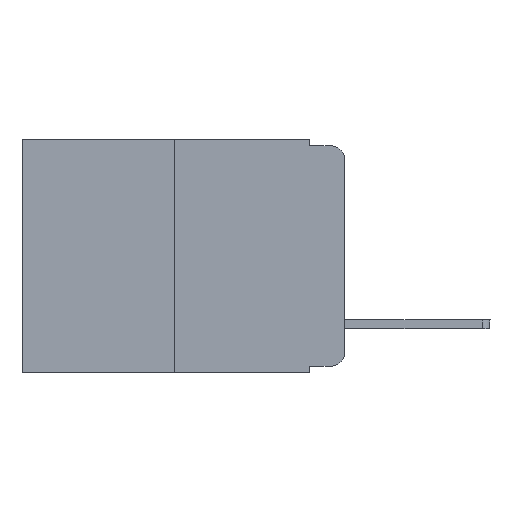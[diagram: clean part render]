
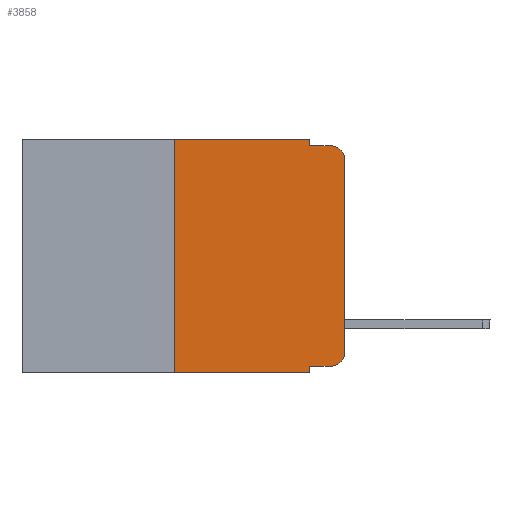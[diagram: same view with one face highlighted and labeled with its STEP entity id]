
A CAD part, left-side view. The second image highlights one B-rep face of the part: STEP entity #3858.
In plain terms, the highlighted planar face has unit normal (-1, 0, 0).
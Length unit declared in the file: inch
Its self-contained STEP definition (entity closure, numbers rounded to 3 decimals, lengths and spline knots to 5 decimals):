
#132 = CARTESIAN_POINT ( 'NONE',  ( 0., 0.473, 0. ) ) ;
#944 = VERTEX_POINT ( 'NONE', #8433 ) ;
#1011 = DIRECTION ( 'NONE',  ( 0., -1., 0. ) ) ;
#1260 = EDGE_CURVE ( 'NONE', #11371, #9000, #10888, .T. ) ;
#1627 = LINE ( 'NONE', #14603, #9006 ) ;
#2044 = CARTESIAN_POINT ( 'NONE',  ( 0., 0., 0. ) ) ;
#2424 = EDGE_CURVE ( 'NONE', #6931, #944, #11698, .T. ) ;
#2818 = DIRECTION ( 'NONE',  ( 0., 0., -1. ) ) ;
#2819 = EDGE_CURVE ( 'NONE', #20794, #2828, #19804, .T. ) ;
#2828 = VERTEX_POINT ( 'NONE', #12035 ) ;
#2847 = CARTESIAN_POINT ( 'NONE',  ( 0., 0.473, 0. ) ) ;
#3095 = VERTEX_POINT ( 'NONE', #4693 ) ;
#3801 = CIRCLE ( 'NONE', #15693, 0.02 ) ;
#3858 = ADVANCED_FACE ( 'NONE', ( #19489 ), #4544, .F. ) ;
#4072 = ORIENTED_EDGE ( 'NONE', *, *, #19238, .F. ) ;
#4544 = PLANE ( 'NONE',  #5736 ) ;
#4693 = CARTESIAN_POINT ( 'NONE',  ( 0., 0., -0.03 ) ) ;
#5736 = AXIS2_PLACEMENT_3D ( 'NONE', #2847, #11032, #18995 ) ;
#6109 = EDGE_CURVE ( 'NONE', #7393, #11371, #6522, .T. ) ;
#6522 = LINE ( 'NONE', #132, #11937 ) ;
#6528 = CARTESIAN_POINT ( 'NONE',  ( 0., 0.051, 0. ) ) ;
#6931 = VERTEX_POINT ( 'NONE', #12402 ) ;
#7074 = CARTESIAN_POINT ( 'NONE',  ( 0., 0.473, -0.343 ) ) ;
#7168 = ORIENTED_EDGE ( 'NONE', *, *, #2819, .F. ) ;
#7237 = EDGE_CURVE ( 'NONE', #20794, #6931, #19071, .T. ) ;
#7270 = CARTESIAN_POINT ( 'NONE',  ( 0., 0.02, -0.313 ) ) ;
#7393 = VERTEX_POINT ( 'NONE', #9703 ) ;
#7691 = CARTESIAN_POINT ( 'NONE',  ( 0., 0.051, -0.333 ) ) ;
#8042 = ORIENTED_EDGE ( 'NONE', *, *, #7237, .T. ) ;
#8433 = CARTESIAN_POINT ( 'NONE',  ( 0., 0., -0.313 ) ) ;
#8497 = LINE ( 'NONE', #2044, #17608 ) ;
#8700 = ORIENTED_EDGE ( 'NONE', *, *, #1260, .F. ) ;
#9000 = VERTEX_POINT ( 'NONE', #17249 ) ;
#9006 = VECTOR ( 'NONE', #11193, 39.37008 ) ;
#9165 = DIRECTION ( 'NONE',  ( 0., -1., 0. ) ) ;
#9703 = CARTESIAN_POINT ( 'NONE',  ( 0., 0.25, 0. ) ) ;
#10057 = CARTESIAN_POINT ( 'NONE',  ( 0., 0.051, 0. ) ) ;
#10234 = LINE ( 'NONE', #16837, #14738 ) ;
#10485 = CARTESIAN_POINT ( 'NONE',  ( 0., 0.02, -0.03 ) ) ;
#10642 = DIRECTION ( 'NONE',  ( 0., 0., 1. ) ) ;
#10888 = LINE ( 'NONE', #6528, #15079 ) ;
#10910 = ORIENTED_EDGE ( 'NONE', *, *, #13569, .F. ) ;
#10985 = ORIENTED_EDGE ( 'NONE', *, *, #2424, .T. ) ;
#11032 = DIRECTION ( 'NONE',  ( 1., 0., 0. ) ) ;
#11193 = DIRECTION ( 'NONE',  ( 0., -1., 0. ) ) ;
#11196 = DIRECTION ( 'NONE',  ( 0., -1., 0. ) ) ;
#11214 = DIRECTION ( 'NONE',  ( 0., 0., 1. ) ) ;
#11371 = VERTEX_POINT ( 'NONE', #10057 ) ;
#11521 = VECTOR ( 'NONE', #9165, 39.37008 ) ;
#11698 = CIRCLE ( 'NONE', #17137, 0.02 ) ;
#11764 = EDGE_CURVE ( 'NONE', #944, #3095, #8497, .T. ) ;
#11937 = VECTOR ( 'NONE', #11196, 39.37008 ) ;
#12035 = CARTESIAN_POINT ( 'NONE',  ( 0., 0.051, -0.343 ) ) ;
#12331 = VECTOR ( 'NONE', #1011, 39.37008 ) ;
#12402 = CARTESIAN_POINT ( 'NONE',  ( 0., 0.02, -0.333 ) ) ;
#12556 = VECTOR ( 'NONE', #20019, 39.37008 ) ;
#12571 = CARTESIAN_POINT ( 'NONE',  ( 0., 0.02, -0.01 ) ) ;
#13373 = DIRECTION ( 'NONE',  ( -1., 0., 0. ) ) ;
#13535 = CARTESIAN_POINT ( 'NONE',  ( 0., 0.051, 0. ) ) ;
#13569 = EDGE_CURVE ( 'NONE', #9000, #19356, #1627, .T. ) ;
#13873 = VERTEX_POINT ( 'NONE', #14480 ) ;
#14063 = CARTESIAN_POINT ( 'NONE',  ( 0., 0.051, -0.333 ) ) ;
#14235 = ORIENTED_EDGE ( 'NONE', *, *, #11764, .T. ) ;
#14480 = CARTESIAN_POINT ( 'NONE',  ( 0., 0.25, -0.343 ) ) ;
#14603 = CARTESIAN_POINT ( 'NONE',  ( 0., 0.051, -0.01 ) ) ;
#14738 = VECTOR ( 'NONE', #10642, 39.37008 ) ;
#15077 = DIRECTION ( 'NONE',  ( 0., 0., -1. ) ) ;
#15079 = VECTOR ( 'NONE', #17378, 39.37008 ) ;
#15693 = AXIS2_PLACEMENT_3D ( 'NONE', #10485, #13373, #15077 ) ;
#15780 = EDGE_CURVE ( 'NONE', #3095, #19356, #3801, .T. ) ;
#16295 = EDGE_LOOP ( 'NONE', ( #14235, #18661, #10910, #8700, #19774, #4072, #17732, #7168, #8042, #10985 ) ) ;
#16837 = CARTESIAN_POINT ( 'NONE',  ( 0., 0.25, 0. ) ) ;
#16962 = LINE ( 'NONE', #7074, #12331 ) ;
#17137 = AXIS2_PLACEMENT_3D ( 'NONE', #7270, #17274, #2818 ) ;
#17249 = CARTESIAN_POINT ( 'NONE',  ( 0., 0.051, -0.01 ) ) ;
#17274 = DIRECTION ( 'NONE',  ( -1., 0., 0. ) ) ;
#17378 = DIRECTION ( 'NONE',  ( 0., 0., -1. ) ) ;
#17608 = VECTOR ( 'NONE', #11214, 39.37008 ) ;
#17732 = ORIENTED_EDGE ( 'NONE', *, *, #18692, .T. ) ;
#18661 = ORIENTED_EDGE ( 'NONE', *, *, #15780, .T. ) ;
#18692 = EDGE_CURVE ( 'NONE', #13873, #2828, #16962, .T. ) ;
#18995 = DIRECTION ( 'NONE',  ( 0., 0., -1. ) ) ;
#19071 = LINE ( 'NONE', #7691, #11521 ) ;
#19238 = EDGE_CURVE ( 'NONE', #13873, #7393, #10234, .T. ) ;
#19356 = VERTEX_POINT ( 'NONE', #12571 ) ;
#19489 = FACE_OUTER_BOUND ( 'NONE', #16295, .T. ) ;
#19774 = ORIENTED_EDGE ( 'NONE', *, *, #6109, .F. ) ;
#19804 = LINE ( 'NONE', #13535, #12556 ) ;
#20019 = DIRECTION ( 'NONE',  ( 0., 0., -1. ) ) ;
#20794 = VERTEX_POINT ( 'NONE', #14063 ) ;
